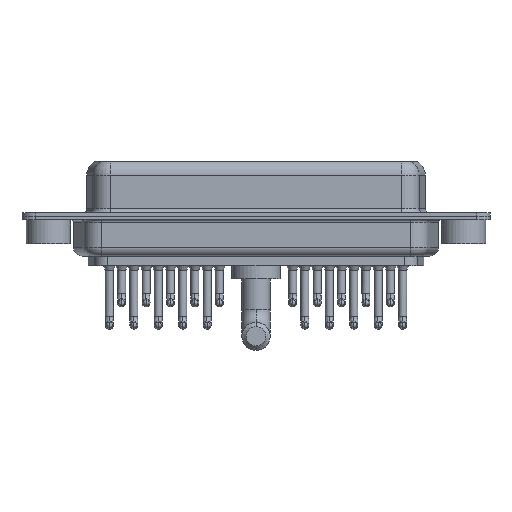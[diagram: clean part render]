
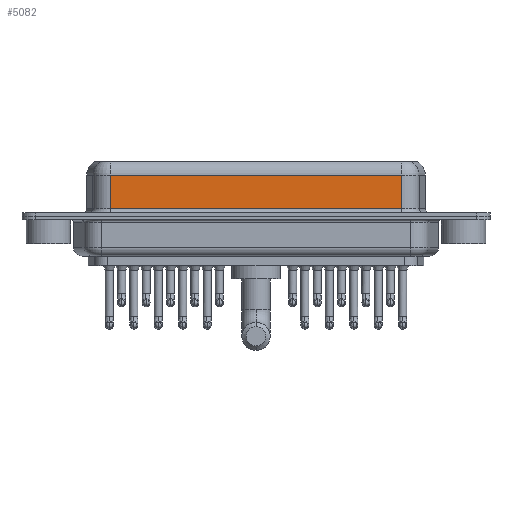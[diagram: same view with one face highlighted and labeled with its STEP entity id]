
A CAD part, front view. The second image highlights one B-rep face of the part: STEP entity #5082.
In plain terms, the highlighted planar face has unit normal (0, -1, 0).
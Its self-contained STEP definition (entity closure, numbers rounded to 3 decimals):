
#283 = CARTESIAN_POINT ( 'NONE',  ( 40.037, -3.95, 6.4 ) ) ;
#675 = VECTOR ( 'NONE', #12765, 1000. ) ;
#865 = AXIS2_PLACEMENT_3D ( 'NONE', #12112, #6739, #17365 ) ;
#1260 = VECTOR ( 'NONE', #20522, 1000. ) ;
#2395 = CARTESIAN_POINT ( 'NONE',  ( 7.013, -3.95, 0.9 ) ) ;
#2729 = CARTESIAN_POINT ( 'NONE',  ( 7.013, -3.95, 6.4 ) ) ;
#3158 = EDGE_CURVE ( 'NONE', #6357, #15910, #16697, .T. ) ;
#3521 = VECTOR ( 'NONE', #14722, 1000. ) ;
#3732 = ORIENTED_EDGE ( 'NONE', *, *, #3885, .T. ) ;
#3885 = EDGE_CURVE ( 'NONE', #9300, #6357, #9782, .T. ) ;
#5082 = ADVANCED_FACE ( 'NONE', ( #15428 ), #22413, .F. ) ;
#6357 = VERTEX_POINT ( 'NONE', #17887 ) ;
#6739 = DIRECTION ( 'NONE',  ( 0., 1., 0. ) ) ;
#6754 = ORIENTED_EDGE ( 'NONE', *, *, #13783, .F. ) ;
#8557 = VECTOR ( 'NONE', #14880, 1000. ) ;
#9300 = VERTEX_POINT ( 'NONE', #20856 ) ;
#9782 = LINE ( 'NONE', #13419, #1260 ) ;
#10946 = LINE ( 'NONE', #283, #675 ) ;
#11466 = ORIENTED_EDGE ( 'NONE', *, *, #3158, .T. ) ;
#11605 = LINE ( 'NONE', #18586, #3521 ) ;
#12112 = CARTESIAN_POINT ( 'NONE',  ( 40.037, -3.95, 6.4 ) ) ;
#12647 = EDGE_CURVE ( 'NONE', #15910, #22494, #11605, .T. ) ;
#12765 = DIRECTION ( 'NONE',  ( 0., 0., -1. ) ) ;
#13419 = CARTESIAN_POINT ( 'NONE',  ( 40.037, -3.95, 4.65 ) ) ;
#13783 = EDGE_CURVE ( 'NONE', #9300, #22494, #10946, .T. ) ;
#14722 = DIRECTION ( 'NONE',  ( 1., 0., 0. ) ) ;
#14880 = DIRECTION ( 'NONE',  ( 0., 0., -1. ) ) ;
#15428 = FACE_OUTER_BOUND ( 'NONE', #18766, .T. ) ;
#15910 = VERTEX_POINT ( 'NONE', #2395 ) ;
#16507 = ORIENTED_EDGE ( 'NONE', *, *, #12647, .T. ) ;
#16697 = LINE ( 'NONE', #2729, #8557 ) ;
#17365 = DIRECTION ( 'NONE',  ( 0., 0., 1. ) ) ;
#17887 = CARTESIAN_POINT ( 'NONE',  ( 7.013, -3.95, 4.65 ) ) ;
#18586 = CARTESIAN_POINT ( 'NONE',  ( 40.037, -3.95, 0.9 ) ) ;
#18766 = EDGE_LOOP ( 'NONE', ( #6754, #3732, #11466, #16507 ) ) ;
#20343 = CARTESIAN_POINT ( 'NONE',  ( 40.037, -3.95, 0.9 ) ) ;
#20522 = DIRECTION ( 'NONE',  ( -1., 0., 0. ) ) ;
#20856 = CARTESIAN_POINT ( 'NONE',  ( 40.037, -3.95, 4.65 ) ) ;
#22413 = PLANE ( 'NONE',  #865 ) ;
#22494 = VERTEX_POINT ( 'NONE', #20343 ) ;
